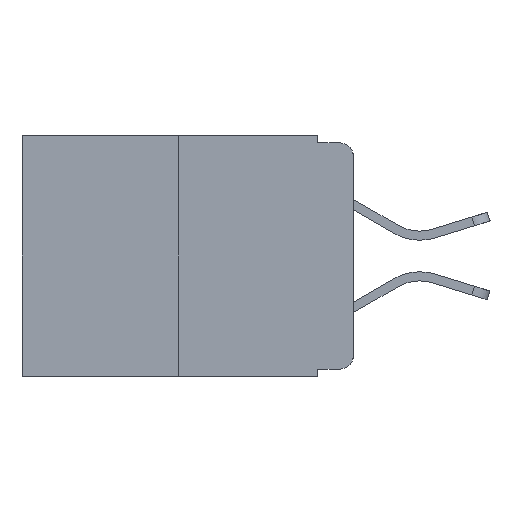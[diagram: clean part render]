
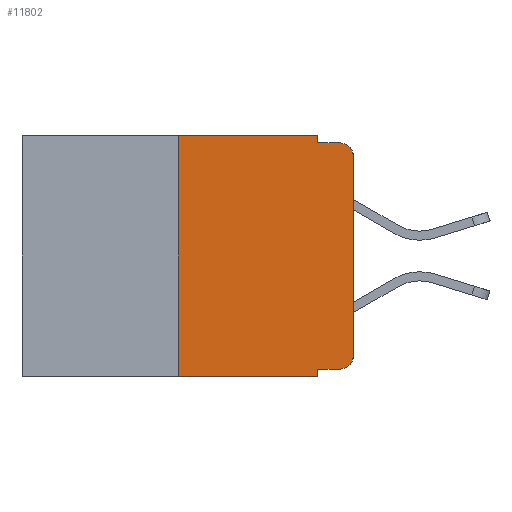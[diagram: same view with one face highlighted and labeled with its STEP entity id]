
A CAD part, left-side view. The second image highlights one B-rep face of the part: STEP entity #11802.
In plain terms, the highlighted planar face has unit normal (-1, 0, 0).
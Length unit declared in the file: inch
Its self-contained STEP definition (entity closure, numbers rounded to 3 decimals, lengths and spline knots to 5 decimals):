
#294 = CARTESIAN_POINT ( 'NONE',  ( 0., 0.25, 0. ) ) ;
#520 = VECTOR ( 'NONE', #21433, 39.37008 ) ;
#754 = EDGE_CURVE ( 'NONE', #1871, #19246, #3048, .T. ) ;
#775 = LINE ( 'NONE', #18109, #1323 ) ;
#1323 = VECTOR ( 'NONE', #9627, 39.37008 ) ;
#1524 = DIRECTION ( 'NONE',  ( 0., 0., 1. ) ) ;
#1816 = CARTESIAN_POINT ( 'NONE',  ( 0., 0.02, -0.313 ) ) ;
#1871 = VERTEX_POINT ( 'NONE', #12549 ) ;
#1944 = EDGE_CURVE ( 'NONE', #13548, #1871, #16337, .T. ) ;
#2915 = VECTOR ( 'NONE', #15291, 39.37008 ) ;
#3048 = CIRCLE ( 'NONE', #3701, 0.02 ) ;
#3701 = AXIS2_PLACEMENT_3D ( 'NONE', #1816, #17349, #17307 ) ;
#4224 = EDGE_CURVE ( 'NONE', #13548, #14926, #20546, .T. ) ;
#4776 = CARTESIAN_POINT ( 'NONE',  ( 0., 0.051, -0.01 ) ) ;
#4879 = VECTOR ( 'NONE', #8300, 39.37008 ) ;
#5582 = ORIENTED_EDGE ( 'NONE', *, *, #12584, .T. ) ;
#5612 = CARTESIAN_POINT ( 'NONE',  ( 0., 0.051, -0.01 ) ) ;
#5658 = LINE ( 'NONE', #19770, #520 ) ;
#6733 = EDGE_CURVE ( 'NONE', #22104, #19371, #9478, .T. ) ;
#6776 = CARTESIAN_POINT ( 'NONE',  ( 0., 0.051, -0.333 ) ) ;
#6991 = DIRECTION ( 'NONE',  ( 1., 0., 0. ) ) ;
#7052 = CARTESIAN_POINT ( 'NONE',  ( 0., 0.051, -0.343 ) ) ;
#7735 = EDGE_CURVE ( 'NONE', #20238, #22104, #13190, .T. ) ;
#7738 = ORIENTED_EDGE ( 'NONE', *, *, #12294, .T. ) ;
#8043 = ORIENTED_EDGE ( 'NONE', *, *, #10023, .F. ) ;
#8280 = ORIENTED_EDGE ( 'NONE', *, *, #11151, .F. ) ;
#8288 = CARTESIAN_POINT ( 'NONE',  ( 0., 0.051, 0. ) ) ;
#8300 = DIRECTION ( 'NONE',  ( 0., -1., 0. ) ) ;
#8328 = VECTOR ( 'NONE', #15827, 39.37008 ) ;
#8336 = CARTESIAN_POINT ( 'NONE',  ( 0., 0., -0.03 ) ) ;
#8490 = CARTESIAN_POINT ( 'NONE',  ( 0., 0.051, 0. ) ) ;
#8859 = ORIENTED_EDGE ( 'NONE', *, *, #1944, .T. ) ;
#9163 = VERTEX_POINT ( 'NONE', #4776 ) ;
#9478 = LINE ( 'NONE', #21764, #4879 ) ;
#9627 = DIRECTION ( 'NONE',  ( 0., 0., 1. ) ) ;
#9752 = CIRCLE ( 'NONE', #10782, 0.02 ) ;
#10023 = EDGE_CURVE ( 'NONE', #19371, #9163, #5658, .T. ) ;
#10113 = CARTESIAN_POINT ( 'NONE',  ( 0., 0.02, -0.03 ) ) ;
#10782 = AXIS2_PLACEMENT_3D ( 'NONE', #10113, #21957, #11824 ) ;
#11151 = EDGE_CURVE ( 'NONE', #9163, #11247, #17902, .T. ) ;
#11247 = VERTEX_POINT ( 'NONE', #14444 ) ;
#11407 = CARTESIAN_POINT ( 'NONE',  ( 0., 0., -0.313 ) ) ;
#11802 = ADVANCED_FACE ( 'NONE', ( #15850 ), #15454, .F. ) ;
#11824 = DIRECTION ( 'NONE',  ( 0., 0., -1. ) ) ;
#11840 = CARTESIAN_POINT ( 'NONE',  ( 0., 0.25, 0. ) ) ;
#12035 = CARTESIAN_POINT ( 'NONE',  ( 0., 0.25, -0.343 ) ) ;
#12280 = VERTEX_POINT ( 'NONE', #8336 ) ;
#12294 = EDGE_CURVE ( 'NONE', #12280, #11247, #9752, .T. ) ;
#12480 = CARTESIAN_POINT ( 'NONE',  ( 0., 0.473, -0.343 ) ) ;
#12549 = CARTESIAN_POINT ( 'NONE',  ( 0., 0.02, -0.333 ) ) ;
#12584 = EDGE_CURVE ( 'NONE', #20238, #14926, #17456, .T. ) ;
#12922 = VECTOR ( 'NONE', #14184, 39.37008 ) ;
#13190 = LINE ( 'NONE', #11840, #21642 ) ;
#13448 = EDGE_CURVE ( 'NONE', #19246, #12280, #775, .T. ) ;
#13548 = VERTEX_POINT ( 'NONE', #6776 ) ;
#14152 = ORIENTED_EDGE ( 'NONE', *, *, #7735, .F. ) ;
#14184 = DIRECTION ( 'NONE',  ( 0., -1., 0. ) ) ;
#14444 = CARTESIAN_POINT ( 'NONE',  ( 0., 0.02, -0.01 ) ) ;
#14484 = CARTESIAN_POINT ( 'NONE',  ( 0., 0.051, -0.333 ) ) ;
#14926 = VERTEX_POINT ( 'NONE', #7052 ) ;
#15201 = ORIENTED_EDGE ( 'NONE', *, *, #4224, .F. ) ;
#15286 = VECTOR ( 'NONE', #17838, 39.37008 ) ;
#15291 = DIRECTION ( 'NONE',  ( 0., 0., -1. ) ) ;
#15450 = ORIENTED_EDGE ( 'NONE', *, *, #13448, .T. ) ;
#15454 = PLANE ( 'NONE',  #19622 ) ;
#15827 = DIRECTION ( 'NONE',  ( 0., -1., 0. ) ) ;
#15850 = FACE_OUTER_BOUND ( 'NONE', #16707, .T. ) ;
#16337 = LINE ( 'NONE', #14484, #15286 ) ;
#16707 = EDGE_LOOP ( 'NONE', ( #15450, #7738, #8280, #8043, #22081, #14152, #5582, #15201, #8859, #17893 ) ) ;
#17201 = CARTESIAN_POINT ( 'NONE',  ( 0., 0.473, 0. ) ) ;
#17307 = DIRECTION ( 'NONE',  ( 0., 0., -1. ) ) ;
#17349 = DIRECTION ( 'NONE',  ( -1., 0., 0. ) ) ;
#17456 = LINE ( 'NONE', #12480, #12922 ) ;
#17838 = DIRECTION ( 'NONE',  ( 0., -1., 0. ) ) ;
#17893 = ORIENTED_EDGE ( 'NONE', *, *, #754, .T. ) ;
#17902 = LINE ( 'NONE', #5612, #8328 ) ;
#18109 = CARTESIAN_POINT ( 'NONE',  ( 0., 0., 0. ) ) ;
#18927 = DIRECTION ( 'NONE',  ( 0., 0., -1. ) ) ;
#19246 = VERTEX_POINT ( 'NONE', #11407 ) ;
#19371 = VERTEX_POINT ( 'NONE', #8288 ) ;
#19622 = AXIS2_PLACEMENT_3D ( 'NONE', #17201, #6991, #18927 ) ;
#19770 = CARTESIAN_POINT ( 'NONE',  ( 0., 0.051, 0. ) ) ;
#20238 = VERTEX_POINT ( 'NONE', #12035 ) ;
#20546 = LINE ( 'NONE', #8490, #2915 ) ;
#21433 = DIRECTION ( 'NONE',  ( 0., 0., -1. ) ) ;
#21642 = VECTOR ( 'NONE', #1524, 39.37008 ) ;
#21764 = CARTESIAN_POINT ( 'NONE',  ( 0., 0.473, 0. ) ) ;
#21957 = DIRECTION ( 'NONE',  ( -1., 0., 0. ) ) ;
#22081 = ORIENTED_EDGE ( 'NONE', *, *, #6733, .F. ) ;
#22104 = VERTEX_POINT ( 'NONE', #294 ) ;
